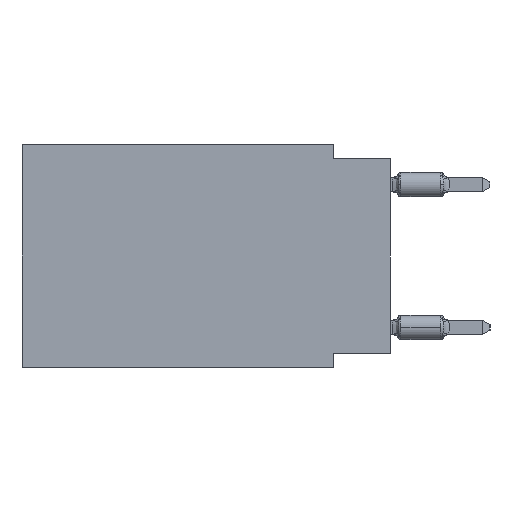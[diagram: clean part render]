
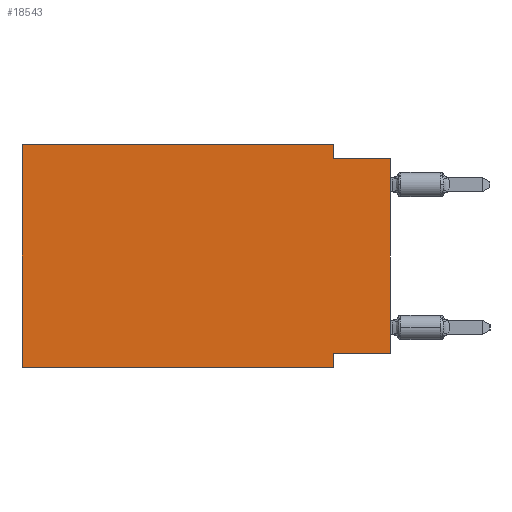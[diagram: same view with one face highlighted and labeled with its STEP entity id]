
A CAD part, left-side view. The second image highlights one B-rep face of the part: STEP entity #18543.
In plain terms, the highlighted planar face has unit normal (-1, 0, 0).
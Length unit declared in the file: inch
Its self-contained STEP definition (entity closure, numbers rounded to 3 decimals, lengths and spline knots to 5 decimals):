
#196 = VECTOR ( 'NONE', #22258, 39.37008 ) ;
#748 = VERTEX_POINT ( 'NONE', #8084 ) ;
#950 = VECTOR ( 'NONE', #14387, 39.37008 ) ;
#1147 = VERTEX_POINT ( 'NONE', #2424 ) ;
#1205 = LINE ( 'NONE', #11864, #196 ) ;
#1716 = LINE ( 'NONE', #19183, #7447 ) ;
#1840 = VECTOR ( 'NONE', #5839, 39.37008 ) ;
#1982 = CARTESIAN_POINT ( 'NONE',  ( 0., 0.645, 0. ) ) ;
#2039 = CARTESIAN_POINT ( 'NONE',  ( 0., 0.1, -0.365 ) ) ;
#2346 = AXIS2_PLACEMENT_3D ( 'NONE', #5072, #16653, #6594 ) ;
#2424 = CARTESIAN_POINT ( 'NONE',  ( 0., 0., -0.025 ) ) ;
#2630 = PLANE ( 'NONE',  #2346 ) ;
#2746 = ORIENTED_EDGE ( 'NONE', *, *, #6458, .F. ) ;
#3865 = EDGE_CURVE ( 'NONE', #9073, #20890, #1205, .T. ) ;
#3898 = EDGE_CURVE ( 'NONE', #748, #9073, #7480, .T. ) ;
#4866 = ORIENTED_EDGE ( 'NONE', *, *, #3898, .F. ) ;
#4890 = EDGE_CURVE ( 'NONE', #21407, #21115, #12354, .T. ) ;
#5072 = CARTESIAN_POINT ( 'NONE',  ( 0., 0.645, 0. ) ) ;
#5418 = CARTESIAN_POINT ( 'NONE',  ( 0., 0.645, 0. ) ) ;
#5839 = DIRECTION ( 'NONE',  ( 0., 0., -1. ) ) ;
#6090 = CARTESIAN_POINT ( 'NONE',  ( 0., 0.1, -0.025 ) ) ;
#6271 = ORIENTED_EDGE ( 'NONE', *, *, #9326, .F. ) ;
#6458 = EDGE_CURVE ( 'NONE', #21115, #17533, #9255, .T. ) ;
#6594 = DIRECTION ( 'NONE',  ( 0., 0., -1. ) ) ;
#7447 = VECTOR ( 'NONE', #10657, 39.37008 ) ;
#7480 = LINE ( 'NONE', #5418, #950 ) ;
#7554 = CARTESIAN_POINT ( 'NONE',  ( 0., 0.1, -0.39 ) ) ;
#7738 = EDGE_CURVE ( 'NONE', #20890, #17913, #21602, .T. ) ;
#8084 = CARTESIAN_POINT ( 'NONE',  ( 0., 0.645, -0.39 ) ) ;
#8092 = ORIENTED_EDGE ( 'NONE', *, *, #7738, .F. ) ;
#8224 = CARTESIAN_POINT ( 'NONE',  ( 0., 0.645, -0.39 ) ) ;
#8425 = VECTOR ( 'NONE', #19056, 39.37008 ) ;
#9073 = VERTEX_POINT ( 'NONE', #1982 ) ;
#9255 = LINE ( 'NONE', #7554, #1840 ) ;
#9326 = EDGE_CURVE ( 'NONE', #17913, #1147, #10385, .T. ) ;
#10040 = ORIENTED_EDGE ( 'NONE', *, *, #3865, .F. ) ;
#10124 = ORIENTED_EDGE ( 'NONE', *, *, #11745, .T. ) ;
#10385 = LINE ( 'NONE', #10862, #14977 ) ;
#10391 = LINE ( 'NONE', #8224, #8425 ) ;
#10657 = DIRECTION ( 'NONE',  ( 0., 0., 1. ) ) ;
#10862 = CARTESIAN_POINT ( 'NONE',  ( 0., 0., -0.025 ) ) ;
#11707 = VECTOR ( 'NONE', #17910, 39.37008 ) ;
#11745 = EDGE_CURVE ( 'NONE', #748, #17533, #10391, .T. ) ;
#11864 = CARTESIAN_POINT ( 'NONE',  ( 0., 0.645, 0. ) ) ;
#11914 = CARTESIAN_POINT ( 'NONE',  ( 0., 0.1, 0. ) ) ;
#12270 = ORIENTED_EDGE ( 'NONE', *, *, #4890, .F. ) ;
#12354 = LINE ( 'NONE', #19378, #14673 ) ;
#14387 = DIRECTION ( 'NONE',  ( 0., 0., 1. ) ) ;
#14394 = CARTESIAN_POINT ( 'NONE',  ( 0., 0.1, -0.39 ) ) ;
#14673 = VECTOR ( 'NONE', #17672, 39.37008 ) ;
#14977 = VECTOR ( 'NONE', #17903, 39.37008 ) ;
#15559 = FACE_OUTER_BOUND ( 'NONE', #21125, .T. ) ;
#16653 = DIRECTION ( 'NONE',  ( 1., 0., 0. ) ) ;
#17533 = VERTEX_POINT ( 'NONE', #14394 ) ;
#17672 = DIRECTION ( 'NONE',  ( 0., 1., 0. ) ) ;
#17903 = DIRECTION ( 'NONE',  ( 0., -1., 0. ) ) ;
#17910 = DIRECTION ( 'NONE',  ( 0., 0., -1. ) ) ;
#17913 = VERTEX_POINT ( 'NONE', #6090 ) ;
#18213 = EDGE_CURVE ( 'NONE', #21407, #1147, #1716, .T. ) ;
#18543 = ADVANCED_FACE ( 'NONE', ( #15559 ), #2630, .F. ) ;
#19056 = DIRECTION ( 'NONE',  ( 0., -1., 0. ) ) ;
#19183 = CARTESIAN_POINT ( 'NONE',  ( 0., 0., 0. ) ) ;
#19378 = CARTESIAN_POINT ( 'NONE',  ( 0., 0., -0.365 ) ) ;
#20528 = ORIENTED_EDGE ( 'NONE', *, *, #18213, .T. ) ;
#20809 = CARTESIAN_POINT ( 'NONE',  ( 0., 0.1, 0. ) ) ;
#20890 = VERTEX_POINT ( 'NONE', #11914 ) ;
#21103 = CARTESIAN_POINT ( 'NONE',  ( 0., 0., -0.365 ) ) ;
#21115 = VERTEX_POINT ( 'NONE', #2039 ) ;
#21125 = EDGE_LOOP ( 'NONE', ( #20528, #6271, #8092, #10040, #4866, #10124, #2746, #12270 ) ) ;
#21407 = VERTEX_POINT ( 'NONE', #21103 ) ;
#21602 = LINE ( 'NONE', #20809, #11707 ) ;
#22258 = DIRECTION ( 'NONE',  ( 0., -1., 0. ) ) ;
